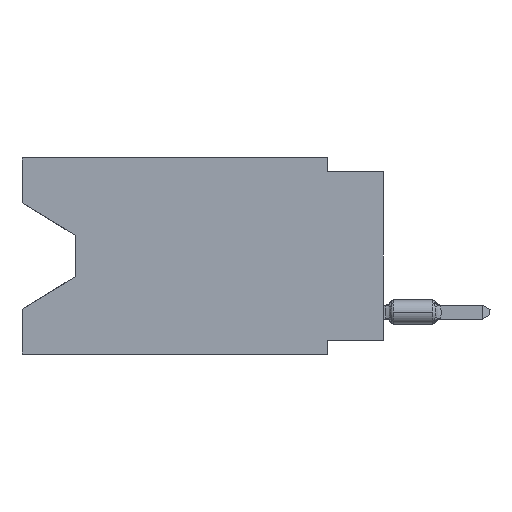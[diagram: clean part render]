
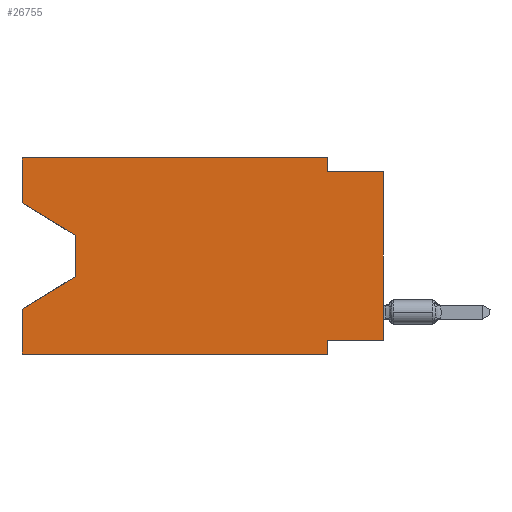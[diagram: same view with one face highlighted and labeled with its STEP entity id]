
A CAD part, left-side view. The second image highlights one B-rep face of the part: STEP entity #26755.
In plain terms, the highlighted planar face has unit normal (-1, 0, 0).
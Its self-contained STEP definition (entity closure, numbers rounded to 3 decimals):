
#416 = VERTEX_POINT ( 'NONE', #40763 ) ;
#610 = LINE ( 'NONE', #13147, #7617 ) ;
#793 = CARTESIAN_POINT ( 'NONE',  ( 0., 2.54, -0.635 ) ) ;
#1075 = EDGE_LOOP ( 'NONE', ( #33524, #7559, #9555, #25890, #8015, #16402, #6824, #41301, #11021, #40212, #39417, #39423 ) ) ;
#1138 = LINE ( 'NONE', #39388, #23255 ) ;
#1392 = VECTOR ( 'NONE', #12195, 1000. ) ;
#1504 = EDGE_CURVE ( 'NONE', #30162, #38559, #4439, .T. ) ;
#2049 = EDGE_CURVE ( 'NONE', #6710, #29993, #14422, .T. ) ;
#3477 = PLANE ( 'NONE',  #5223 ) ;
#3667 = EDGE_CURVE ( 'NONE', #18795, #33558, #19267, .T. ) ;
#3694 = CARTESIAN_POINT ( 'NONE',  ( 0., 13.97, -5.385 ) ) ;
#4439 = LINE ( 'NONE', #17208, #13101 ) ;
#4705 = DIRECTION ( 'NONE',  ( 0., 0., -1. ) ) ;
#4860 = VECTOR ( 'NONE', #37327, 1000. ) ;
#5223 = AXIS2_PLACEMENT_3D ( 'NONE', #16223, #19997, #4705 ) ;
#6626 = CARTESIAN_POINT ( 'NONE',  ( 0., 16.383, -8.89 ) ) ;
#6710 = VERTEX_POINT ( 'NONE', #39704 ) ;
#6788 = LINE ( 'NONE', #13479, #16750 ) ;
#6824 = ORIENTED_EDGE ( 'NONE', *, *, #15041, .F. ) ;
#7559 = ORIENTED_EDGE ( 'NONE', *, *, #2049, .T. ) ;
#7617 = VECTOR ( 'NONE', #13361, 1000. ) ;
#7621 = VECTOR ( 'NONE', #19182, 1000. ) ;
#8015 = ORIENTED_EDGE ( 'NONE', *, *, #36945, .T. ) ;
#8811 = CARTESIAN_POINT ( 'NONE',  ( 0., 16.383, 0. ) ) ;
#9555 = ORIENTED_EDGE ( 'NONE', *, *, #17630, .T. ) ;
#11021 = ORIENTED_EDGE ( 'NONE', *, *, #31609, .F. ) ;
#12195 = DIRECTION ( 'NONE',  ( 0., 1., 0. ) ) ;
#12402 = CARTESIAN_POINT ( 'NONE',  ( 0., 0., -8.255 ) ) ;
#13044 = CARTESIAN_POINT ( 'NONE',  ( 0., 16.383, 0. ) ) ;
#13101 = VECTOR ( 'NONE', #36409, 1000. ) ;
#13147 = CARTESIAN_POINT ( 'NONE',  ( 0., 2.54, 0. ) ) ;
#13189 = VERTEX_POINT ( 'NONE', #34118 ) ;
#13361 = DIRECTION ( 'NONE',  ( 0., 0., -1. ) ) ;
#13479 = CARTESIAN_POINT ( 'NONE',  ( 0., 0., -0.635 ) ) ;
#13895 = DIRECTION ( 'NONE',  ( 0., -0.855, -0.519 ) ) ;
#14422 = LINE ( 'NONE', #24256, #37826 ) ;
#14429 = VERTEX_POINT ( 'NONE', #793 ) ;
#15041 = EDGE_CURVE ( 'NONE', #18795, #18770, #34783, .T. ) ;
#16014 = LINE ( 'NONE', #29170, #36569 ) ;
#16223 = CARTESIAN_POINT ( 'NONE',  ( 0., 16.383, 0. ) ) ;
#16402 = ORIENTED_EDGE ( 'NONE', *, *, #19628, .F. ) ;
#16631 = DIRECTION ( 'NONE',  ( 0., 0.855, -0.519 ) ) ;
#16750 = VECTOR ( 'NONE', #36233, 1000. ) ;
#17208 = CARTESIAN_POINT ( 'NONE',  ( 0., 16.383, 0. ) ) ;
#17630 = EDGE_CURVE ( 'NONE', #29993, #416, #16014, .T. ) ;
#17841 = EDGE_CURVE ( 'NONE', #13189, #6710, #1138, .T. ) ;
#18445 = DIRECTION ( 'NONE',  ( 0., 0., 1. ) ) ;
#18770 = VERTEX_POINT ( 'NONE', #29273 ) ;
#18795 = VERTEX_POINT ( 'NONE', #19667 ) ;
#19182 = DIRECTION ( 'NONE',  ( 0., -1., 0. ) ) ;
#19267 = LINE ( 'NONE', #38872, #39226 ) ;
#19384 = FACE_OUTER_BOUND ( 'NONE', #1075, .T. ) ;
#19628 = EDGE_CURVE ( 'NONE', #18770, #29537, #33154, .T. ) ;
#19667 = CARTESIAN_POINT ( 'NONE',  ( 0., 0., -8.255 ) ) ;
#19997 = DIRECTION ( 'NONE',  ( 1., 0., 0. ) ) ;
#22199 = LINE ( 'NONE', #8811, #29400 ) ;
#23255 = VECTOR ( 'NONE', #13895, 1000. ) ;
#23879 = CARTESIAN_POINT ( 'NONE',  ( 0., 0., -0.635 ) ) ;
#24256 = CARTESIAN_POINT ( 'NONE',  ( 0., 13.97, -3.505 ) ) ;
#24514 = EDGE_CURVE ( 'NONE', #30359, #416, #22199, .T. ) ;
#25324 = DIRECTION ( 'NONE',  ( 0., 0., 1. ) ) ;
#25890 = ORIENTED_EDGE ( 'NONE', *, *, #24514, .F. ) ;
#26755 = ADVANCED_FACE ( 'NONE', ( #19384 ), #3477, .F. ) ;
#28369 = CARTESIAN_POINT ( 'NONE',  ( 0., 2.54, 0. ) ) ;
#28806 = LINE ( 'NONE', #6626, #7621 ) ;
#29170 = CARTESIAN_POINT ( 'NONE',  ( 0., 13.97, -5.385 ) ) ;
#29273 = CARTESIAN_POINT ( 'NONE',  ( 0., 2.54, -8.255 ) ) ;
#29400 = VECTOR ( 'NONE', #18445, 1000. ) ;
#29537 = VERTEX_POINT ( 'NONE', #34712 ) ;
#29993 = VERTEX_POINT ( 'NONE', #3694 ) ;
#30162 = VERTEX_POINT ( 'NONE', #36701 ) ;
#30359 = VERTEX_POINT ( 'NONE', #35825 ) ;
#30675 = CARTESIAN_POINT ( 'NONE',  ( 0., 2.54, -8.89 ) ) ;
#31463 = LINE ( 'NONE', #13044, #41019 ) ;
#31609 = EDGE_CURVE ( 'NONE', #14429, #33558, #6788, .T. ) ;
#33154 = LINE ( 'NONE', #30675, #4860 ) ;
#33524 = ORIENTED_EDGE ( 'NONE', *, *, #17841, .T. ) ;
#33558 = VERTEX_POINT ( 'NONE', #23879 ) ;
#34118 = CARTESIAN_POINT ( 'NONE',  ( 0., 16.383, -2.038 ) ) ;
#34712 = CARTESIAN_POINT ( 'NONE',  ( 0., 2.54, -8.89 ) ) ;
#34783 = LINE ( 'NONE', #12402, #1392 ) ;
#35825 = CARTESIAN_POINT ( 'NONE',  ( 0., 16.383, -8.89 ) ) ;
#36233 = DIRECTION ( 'NONE',  ( 0., -1., 0. ) ) ;
#36409 = DIRECTION ( 'NONE',  ( 0., -1., 0. ) ) ;
#36569 = VECTOR ( 'NONE', #16631, 1000. ) ;
#36701 = CARTESIAN_POINT ( 'NONE',  ( 0., 16.383, 0. ) ) ;
#36945 = EDGE_CURVE ( 'NONE', #30359, #29537, #28806, .T. ) ;
#37327 = DIRECTION ( 'NONE',  ( 0., 0., -1. ) ) ;
#37604 = DIRECTION ( 'NONE',  ( 0., 0., -1. ) ) ;
#37826 = VECTOR ( 'NONE', #37604, 1000. ) ;
#37911 = DIRECTION ( 'NONE',  ( 0., 0., 1. ) ) ;
#38559 = VERTEX_POINT ( 'NONE', #28369 ) ;
#38872 = CARTESIAN_POINT ( 'NONE',  ( 0., 0., 0. ) ) ;
#38990 = EDGE_CURVE ( 'NONE', #13189, #30162, #31463, .T. ) ;
#39226 = VECTOR ( 'NONE', #25324, 1000. ) ;
#39331 = EDGE_CURVE ( 'NONE', #38559, #14429, #610, .T. ) ;
#39388 = CARTESIAN_POINT ( 'NONE',  ( 0., 16.383, -2.038 ) ) ;
#39417 = ORIENTED_EDGE ( 'NONE', *, *, #1504, .F. ) ;
#39423 = ORIENTED_EDGE ( 'NONE', *, *, #38990, .F. ) ;
#39704 = CARTESIAN_POINT ( 'NONE',  ( 0., 13.97, -3.505 ) ) ;
#40212 = ORIENTED_EDGE ( 'NONE', *, *, #39331, .F. ) ;
#40763 = CARTESIAN_POINT ( 'NONE',  ( 0., 16.383, -6.852 ) ) ;
#41019 = VECTOR ( 'NONE', #37911, 1000. ) ;
#41301 = ORIENTED_EDGE ( 'NONE', *, *, #3667, .T. ) ;
